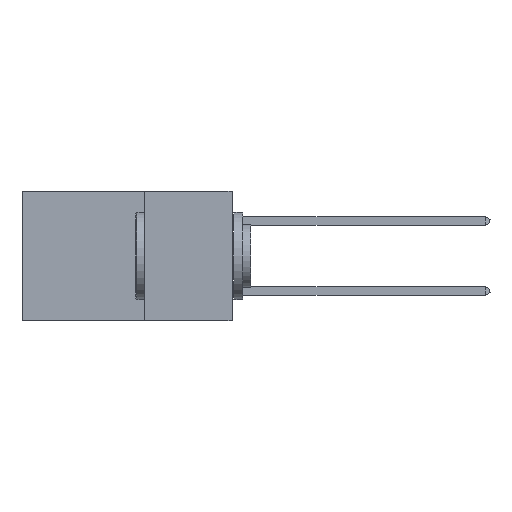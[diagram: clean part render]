
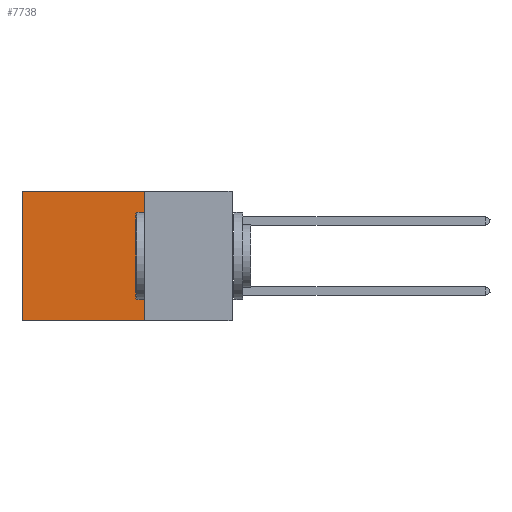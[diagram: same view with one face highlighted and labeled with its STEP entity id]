
A CAD part, left-side view. The second image highlights one B-rep face of the part: STEP entity #7738.
In plain terms, the highlighted planar face has unit normal (-1, 0, 0).
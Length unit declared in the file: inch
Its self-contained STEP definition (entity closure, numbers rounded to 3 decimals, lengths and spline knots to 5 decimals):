
#249 = ORIENTED_EDGE ( 'NONE', *, *, #45623, .F. ) ;
#2090 = CARTESIAN_POINT ( 'NONE',  ( 0.2875, 0.25, -0.37 ) ) ;
#2908 = LINE ( 'NONE', #38455, #30430 ) ;
#6376 = VERTEX_POINT ( 'NONE', #37237 ) ;
#6557 = LINE ( 'NONE', #2090, #25351 ) ;
#7738 = ADVANCED_FACE ( 'NONE', ( #27221 ), #27692, .F. ) ;
#9530 = VERTEX_POINT ( 'NONE', #41485 ) ;
#12971 = DIRECTION ( 'NONE',  ( 1., 0., 0. ) ) ;
#14785 = AXIS2_PLACEMENT_3D ( 'NONE', #34989, #12971, #38639 ) ;
#16278 = VECTOR ( 'NONE', #21546, 39.37008 ) ;
#17640 = EDGE_LOOP ( 'NONE', ( #45454, #37347, #249, #38860 ) ) ;
#19311 = EDGE_CURVE ( 'NONE', #33302, #6376, #2908, .T. ) ;
#21546 = DIRECTION ( 'NONE',  ( 0., 0., -1. ) ) ;
#22941 = CARTESIAN_POINT ( 'NONE',  ( 0.2875, 0.25, 0. ) ) ;
#25351 = VECTOR ( 'NONE', #39281, 39.37008 ) ;
#27221 = FACE_OUTER_BOUND ( 'NONE', #17640, .T. ) ;
#27692 = PLANE ( 'NONE',  #14785 ) ;
#30430 = VECTOR ( 'NONE', #45719, 39.37008 ) ;
#32829 = DIRECTION ( 'NONE',  ( 0., 0., -1. ) ) ;
#33302 = VERTEX_POINT ( 'NONE', #22941 ) ;
#34989 = CARTESIAN_POINT ( 'NONE',  ( 0.2875, 0.25, 0. ) ) ;
#36066 = LINE ( 'NONE', #40087, #37177 ) ;
#36882 = LINE ( 'NONE', #39713, #16278 ) ;
#37177 = VECTOR ( 'NONE', #32829, 39.37008 ) ;
#37228 = EDGE_CURVE ( 'NONE', #6376, #9530, #36066, .T. ) ;
#37237 = CARTESIAN_POINT ( 'NONE',  ( 0.2875, 0.6, 0. ) ) ;
#37347 = ORIENTED_EDGE ( 'NONE', *, *, #40128, .F. ) ;
#38455 = CARTESIAN_POINT ( 'NONE',  ( 0.2875, 0.25, 0. ) ) ;
#38639 = DIRECTION ( 'NONE',  ( 0., 0., -1. ) ) ;
#38860 = ORIENTED_EDGE ( 'NONE', *, *, #19311, .T. ) ;
#39281 = DIRECTION ( 'NONE',  ( 0., 1., 0. ) ) ;
#39713 = CARTESIAN_POINT ( 'NONE',  ( 0.2875, 0.25, 0. ) ) ;
#40087 = CARTESIAN_POINT ( 'NONE',  ( 0.2875, 0.6, 0. ) ) ;
#40128 = EDGE_CURVE ( 'NONE', #40313, #9530, #6557, .T. ) ;
#40313 = VERTEX_POINT ( 'NONE', #44607 ) ;
#41485 = CARTESIAN_POINT ( 'NONE',  ( 0.2875, 0.6, -0.37 ) ) ;
#44607 = CARTESIAN_POINT ( 'NONE',  ( 0.2875, 0.25, -0.37 ) ) ;
#45454 = ORIENTED_EDGE ( 'NONE', *, *, #37228, .T. ) ;
#45623 = EDGE_CURVE ( 'NONE', #33302, #40313, #36882, .T. ) ;
#45719 = DIRECTION ( 'NONE',  ( 0., 1., 0. ) ) ;
